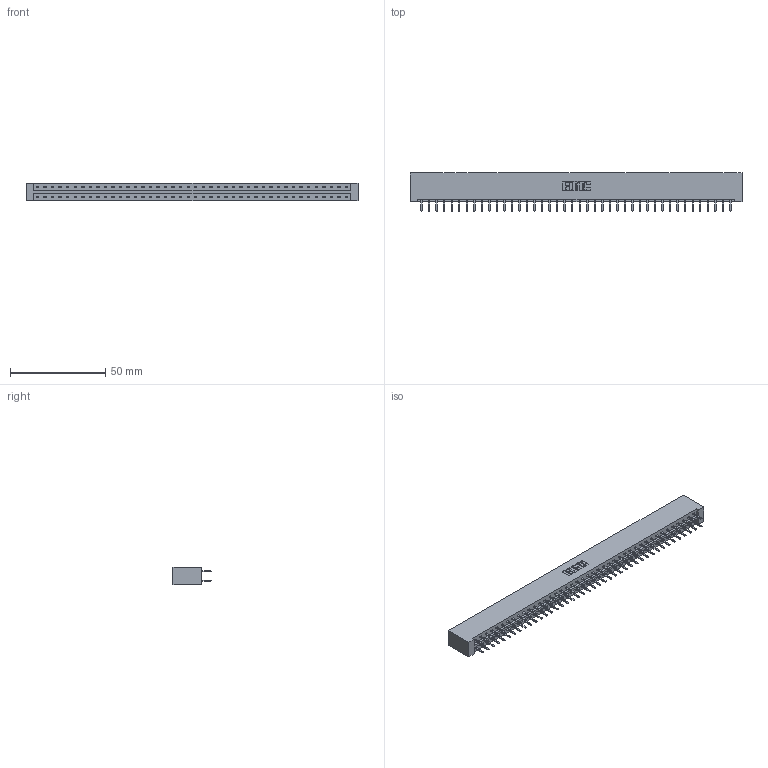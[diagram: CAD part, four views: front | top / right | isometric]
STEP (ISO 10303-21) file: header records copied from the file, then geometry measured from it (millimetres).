
FILE_DESCRIPTION (( 'STEP AP203' ), '1' );
FILE_NAME ('333-084-520-201.STEP', '2018-08-05T04:01:41', ( '' ), ( '' ), 'SwSTEP 2.0', 'SolidWorks 2016', '' );
FILE_SCHEMA (( 'CONFIG_CONTROL_DESIGN' ));
Length unit declared in the file: inch
Products named in the file (3): 333 Part_Lugless; 345-292-001_345-293-120; 333-084-520-201
Assembly tree (85 placements, depth 2):
  333-084-520-201
    333 Part_Lugless
    345-292-001_345-293-120  x84
Bounding box: 174.68 x 20.02 x 9.4 mm (x, y, z)
Volume: 18428.7 mm3; surface area: 21713.9 mm2
Topology: 85 solids, 85 shells, 4810 faces, 13979 edges, 9094 vertices
Faces by surface type: plane 3258, cylinder 1552
Entity records: 26857 total; most frequent: CARTESIAN_POINT 4462, ORIENTED_EDGE 4386, DIRECTION 3793, EDGE_CURVE 2193, VECTOR 2069, LINE 2069, VERTEX_POINT 1458, AXIS2_PLACEMENT_3D 862
